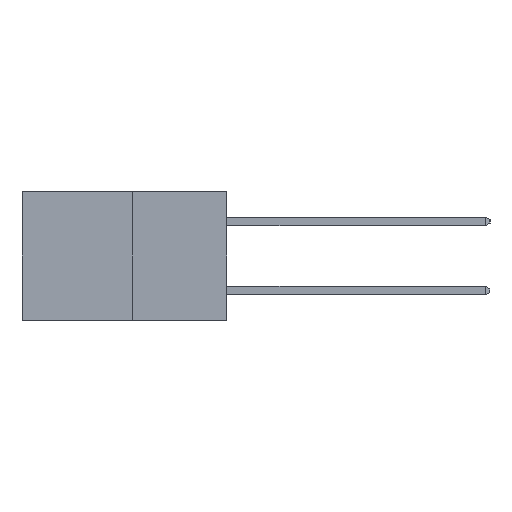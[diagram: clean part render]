
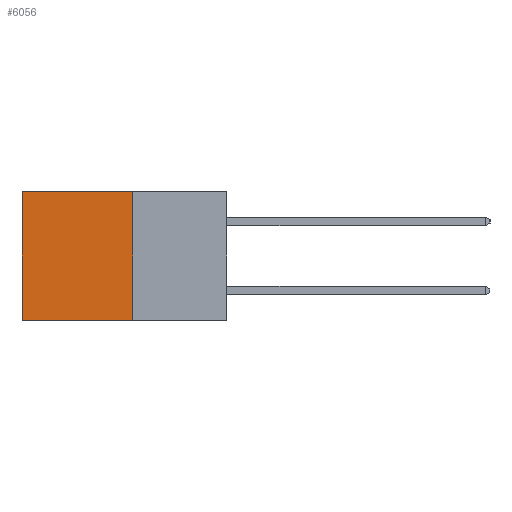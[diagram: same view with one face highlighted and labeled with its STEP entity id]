
A CAD part, left-side view. The second image highlights one B-rep face of the part: STEP entity #6056.
In plain terms, the highlighted planar face has unit normal (-1, 0, 0).
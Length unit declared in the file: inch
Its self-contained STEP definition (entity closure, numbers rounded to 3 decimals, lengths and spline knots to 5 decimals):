
#170 = FACE_OUTER_BOUND ( 'NONE', #5241, .T. ) ;
#199 = VERTEX_POINT ( 'NONE', #9411 ) ;
#284 = PLANE ( 'NONE',  #11288 ) ;
#686 = ORIENTED_EDGE ( 'NONE', *, *, #13425, .F. ) ;
#1034 = LINE ( 'NONE', #9520, #11792 ) ;
#2051 = EDGE_CURVE ( 'NONE', #199, #10774, #10846, .T. ) ;
#2435 = ORIENTED_EDGE ( 'NONE', *, *, #2051, .F. ) ;
#3253 = CARTESIAN_POINT ( 'NONE',  ( 0.277, 0.27, -0.37 ) ) ;
#3594 = CARTESIAN_POINT ( 'NONE',  ( 0.277, 0.27, -0.37 ) ) ;
#4364 = VERTEX_POINT ( 'NONE', #7401 ) ;
#4584 = CARTESIAN_POINT ( 'NONE',  ( 0.277, 0.27, 0. ) ) ;
#5106 = DIRECTION ( 'NONE',  ( 0., 1., 0. ) ) ;
#5241 = EDGE_LOOP ( 'NONE', ( #14926, #2435, #686, #5283 ) ) ;
#5260 = DIRECTION ( 'NONE',  ( 0., 0., -1. ) ) ;
#5283 = ORIENTED_EDGE ( 'NONE', *, *, #7157, .T. ) ;
#6056 = ADVANCED_FACE ( 'NONE', ( #170 ), #284, .F. ) ;
#6783 = CARTESIAN_POINT ( 'NONE',  ( 0.277, 0.59, -0.37 ) ) ;
#6933 = DIRECTION ( 'NONE',  ( 1., 0., 0. ) ) ;
#7026 = DIRECTION ( 'NONE',  ( 0., 0., -1. ) ) ;
#7157 = EDGE_CURVE ( 'NONE', #16343, #4364, #1034, .T. ) ;
#7401 = CARTESIAN_POINT ( 'NONE',  ( 0.277, 0.59, 0. ) ) ;
#9411 = CARTESIAN_POINT ( 'NONE',  ( 0.277, 0.27, -0.37 ) ) ;
#9520 = CARTESIAN_POINT ( 'NONE',  ( 0.277, 0.27, 0. ) ) ;
#10005 = LINE ( 'NONE', #15541, #15991 ) ;
#10219 = DIRECTION ( 'NONE',  ( 0., 1., 0. ) ) ;
#10774 = VERTEX_POINT ( 'NONE', #6783 ) ;
#10846 = LINE ( 'NONE', #3594, #11243 ) ;
#11243 = VECTOR ( 'NONE', #5106, 39.37008 ) ;
#11288 = AXIS2_PLACEMENT_3D ( 'NONE', #12271, #6933, #7026 ) ;
#11792 = VECTOR ( 'NONE', #10219, 39.37008 ) ;
#12271 = CARTESIAN_POINT ( 'NONE',  ( 0.277, 0.27, -0.37 ) ) ;
#13425 = EDGE_CURVE ( 'NONE', #16343, #199, #16022, .T. ) ;
#14926 = ORIENTED_EDGE ( 'NONE', *, *, #14968, .T. ) ;
#14968 = EDGE_CURVE ( 'NONE', #4364, #10774, #10005, .T. ) ;
#14984 = DIRECTION ( 'NONE',  ( 0., 0., -1. ) ) ;
#15541 = CARTESIAN_POINT ( 'NONE',  ( 0.277, 0.59, -0.37 ) ) ;
#15625 = VECTOR ( 'NONE', #14984, 39.37008 ) ;
#15991 = VECTOR ( 'NONE', #5260, 39.37008 ) ;
#16022 = LINE ( 'NONE', #3253, #15625 ) ;
#16343 = VERTEX_POINT ( 'NONE', #4584 ) ;
